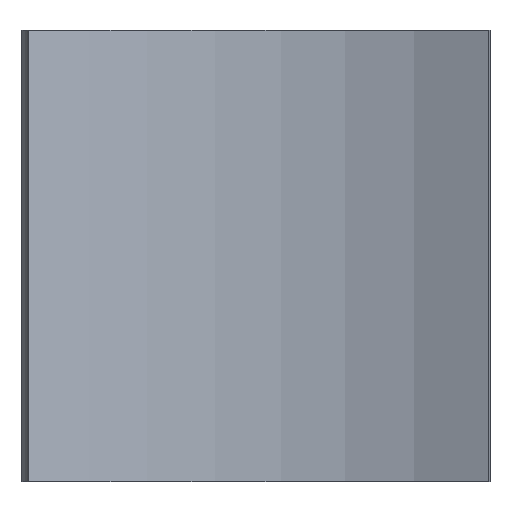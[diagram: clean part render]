
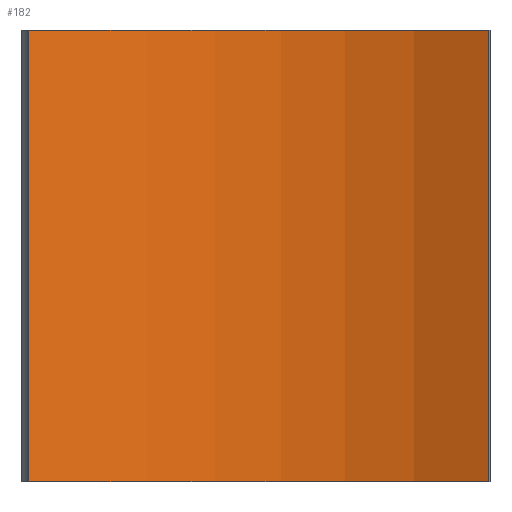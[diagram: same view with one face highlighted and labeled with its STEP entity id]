
A CAD part, front view. The second image highlights one B-rep face of the part: STEP entity #182.
In plain terms, the highlighted free-form (B-spline) face has degree [2, 1] with [3, 2] control points.
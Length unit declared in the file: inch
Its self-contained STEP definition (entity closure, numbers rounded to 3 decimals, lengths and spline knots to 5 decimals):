
#2 = CARTESIAN_POINT ( 'NONE',  ( 23.95857, 0.59599, 0. ) ) ;
#12 = CARTESIAN_POINT ( 'NONE',  ( 19.88297, 0.59889, 4. ) ) ;
#27 = CARTESIAN_POINT ( 'NONE',  ( 19.88297, 0.59889, 4. ) ) ;
#38 = EDGE_CURVE ( 'NONE', #250, #164, #255, .T. ) ;
#51 = B_SPLINE_SURFACE_WITH_KNOTS ( 'NONE', 2, 1, ( 
 ( #66, #2 ),
 ( #56, #252 ),
 ( #165, #115 ) ),
 .UNSPECIFIED., .F., .F., .F.,
 ( 3, 3 ),
 ( 2, 2 ),
 ( 0., 1. ),
 ( 0., 1. ),
 .UNSPECIFIED. ) ;
#54 = EDGE_CURVE ( 'NONE', #342, #250, #235, .T. ) ;
#55 = FACE_OUTER_BOUND ( 'NONE', #180, .T. ) ;
#56 = CARTESIAN_POINT ( 'NONE',  ( 22.12459, 1.58832, 4. ) ) ;
#61 = CARTESIAN_POINT ( 'NONE',  ( 23.95857, 0.59599, 0. ) ) ;
#66 = CARTESIAN_POINT ( 'NONE',  ( 23.95857, 0.59599, 4. ) ) ;
#88 = CARTESIAN_POINT ( 'NONE',  ( 19.88297, 0.59889, 0. ) ) ;
#90 = CARTESIAN_POINT ( 'NONE',  ( 22.12459, 1.58832, 4. ) ) ;
#91 = LINE ( 'NONE', #381, #177 ) ;
#110 = EDGE_CURVE ( 'NONE', #342, #207, #335, .T. ) ;
#115 = CARTESIAN_POINT ( 'NONE',  ( 19.88297, 0.59889, 0. ) ) ;
#124 = ORIENTED_EDGE ( 'NONE', *, *, #110, .T. ) ;
#125 = CARTESIAN_POINT ( 'NONE',  ( 23.95857, 0.59599, 4. ) ) ;
#126 = DIRECTION ( 'NONE',  ( 0., 0., -1. ) ) ;
#130 = CARTESIAN_POINT ( 'NONE',  ( 23.95857, 0.59599, 4. ) ) ;
#164 = VERTEX_POINT ( 'NONE', #88 ) ;
#165 = CARTESIAN_POINT ( 'NONE',  ( 19.88297, 0.59889, 4. ) ) ;
#177 = VECTOR ( 'NONE', #126, 39.37008 ) ;
#180 = EDGE_LOOP ( 'NONE', ( #270, #293, #124, #318 ) ) ;
#182 = ADVANCED_FACE ( 'NONE', ( #55 ), #51, .T. ) ;
#198 = VECTOR ( 'NONE', #202, 39.37008 ) ;
#202 = DIRECTION ( 'NONE',  ( 0., 0., -1. ) ) ;
#203 = CARTESIAN_POINT ( 'NONE',  ( 19.88297, 0.59889, 0. ) ) ;
#207 = VERTEX_POINT ( 'NONE', #27 ) ;
#235 = LINE ( 'NONE', #266, #198 ) ;
#250 = VERTEX_POINT ( 'NONE', #61 ) ;
#252 = CARTESIAN_POINT ( 'NONE',  ( 22.12459, 1.58832, 0. ) ) ;
#255 = B_SPLINE_CURVE_WITH_KNOTS ( 'NONE', 2,
 ( #299, #336, #203 ),
 .UNSPECIFIED., .F., .F.,
 ( 3, 3 ),
 ( 0., 1. ),
 .UNSPECIFIED. ) ;
#266 = CARTESIAN_POINT ( 'NONE',  ( 23.95857, 0.59599, 4. ) ) ;
#270 = ORIENTED_EDGE ( 'NONE', *, *, #38, .F. ) ;
#293 = ORIENTED_EDGE ( 'NONE', *, *, #54, .F. ) ;
#299 = CARTESIAN_POINT ( 'NONE',  ( 23.95857, 0.59599, 0. ) ) ;
#318 = ORIENTED_EDGE ( 'NONE', *, *, #321, .T. ) ;
#321 = EDGE_CURVE ( 'NONE', #207, #164, #91, .T. ) ;
#335 = B_SPLINE_CURVE_WITH_KNOTS ( 'NONE', 2,
 ( #125, #90, #12 ),
 .UNSPECIFIED., .F., .F.,
 ( 3, 3 ),
 ( 0., 1. ),
 .UNSPECIFIED. ) ;
#336 = CARTESIAN_POINT ( 'NONE',  ( 22.12459, 1.58832, 0. ) ) ;
#342 = VERTEX_POINT ( 'NONE', #130 ) ;
#381 = CARTESIAN_POINT ( 'NONE',  ( 19.88297, 0.59889, 4. ) ) ;
